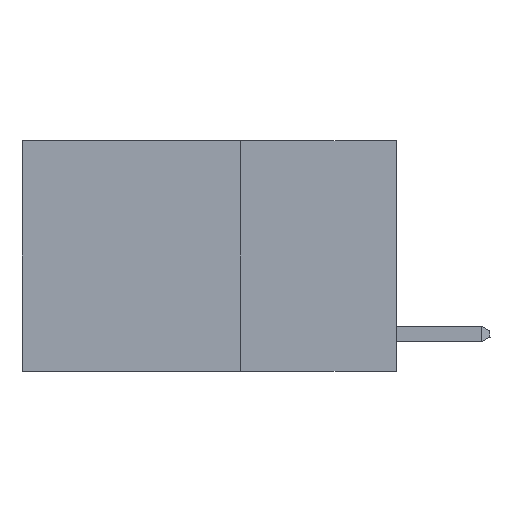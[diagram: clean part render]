
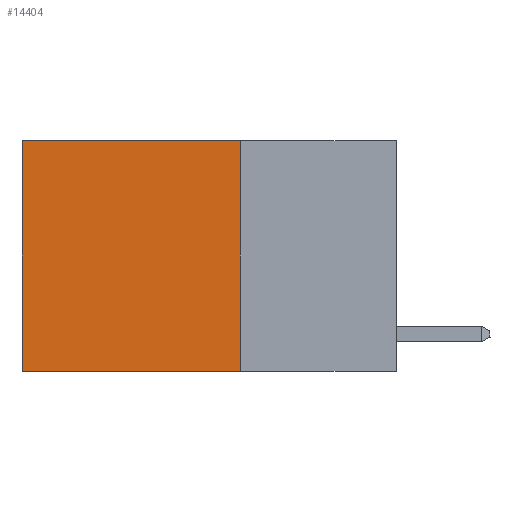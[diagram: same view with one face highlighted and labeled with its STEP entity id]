
A CAD part, left-side view. The second image highlights one B-rep face of the part: STEP entity #14404.
In plain terms, the highlighted planar face has unit normal (-1, 0, 0).
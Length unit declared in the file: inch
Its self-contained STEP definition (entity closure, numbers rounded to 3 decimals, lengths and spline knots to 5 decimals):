
#679 = EDGE_LOOP ( 'NONE', ( #9657, #26297, #12082, #3333 ) ) ;
#1653 = LINE ( 'NONE', #24802, #18273 ) ;
#2124 = VECTOR ( 'NONE', #5819, 39.37008 ) ;
#2194 = CARTESIAN_POINT ( 'NONE',  ( 0.2625, 0.25, 0. ) ) ;
#2763 = LINE ( 'NONE', #22491, #2124 ) ;
#2855 = VERTEX_POINT ( 'NONE', #24447 ) ;
#2958 = EDGE_CURVE ( 'NONE', #21855, #2855, #1653, .T. ) ;
#3333 = ORIENTED_EDGE ( 'NONE', *, *, #18705, .T. ) ;
#3646 = LINE ( 'NONE', #19617, #8541 ) ;
#5655 = EDGE_CURVE ( 'NONE', #2855, #15438, #5745, .T. ) ;
#5745 = LINE ( 'NONE', #22711, #21695 ) ;
#5819 = DIRECTION ( 'NONE',  ( 0., 0., -1. ) ) ;
#6440 = DIRECTION ( 'NONE',  ( 0., 0., -1. ) ) ;
#8541 = VECTOR ( 'NONE', #11299, 39.37008 ) ;
#9657 = ORIENTED_EDGE ( 'NONE', *, *, #17073, .T. ) ;
#11299 = DIRECTION ( 'NONE',  ( 0., 1., 0. ) ) ;
#12082 = ORIENTED_EDGE ( 'NONE', *, *, #2958, .F. ) ;
#12269 = DIRECTION ( 'NONE',  ( 0., 0., -1. ) ) ;
#12712 = CARTESIAN_POINT ( 'NONE',  ( 0.2625, 0.25, 0. ) ) ;
#14404 = ADVANCED_FACE ( 'NONE', ( #15627 ), #16747, .F. ) ;
#15438 = VERTEX_POINT ( 'NONE', #21534 ) ;
#15627 = FACE_OUTER_BOUND ( 'NONE', #679, .T. ) ;
#16358 = DIRECTION ( 'NONE',  ( 0., 1., 0. ) ) ;
#16394 = VERTEX_POINT ( 'NONE', #20496 ) ;
#16747 = PLANE ( 'NONE',  #19987 ) ;
#17073 = EDGE_CURVE ( 'NONE', #16394, #15438, #2763, .T. ) ;
#18273 = VECTOR ( 'NONE', #12269, 39.37008 ) ;
#18705 = EDGE_CURVE ( 'NONE', #21855, #16394, #3646, .T. ) ;
#18878 = DIRECTION ( 'NONE',  ( 1., 0., 0. ) ) ;
#19617 = CARTESIAN_POINT ( 'NONE',  ( 0.2625, 0.25, 0. ) ) ;
#19987 = AXIS2_PLACEMENT_3D ( 'NONE', #2194, #18878, #6440 ) ;
#20496 = CARTESIAN_POINT ( 'NONE',  ( 0.2625, 0.6, 0. ) ) ;
#21534 = CARTESIAN_POINT ( 'NONE',  ( 0.2625, 0.6, -0.37 ) ) ;
#21695 = VECTOR ( 'NONE', #16358, 39.37008 ) ;
#21855 = VERTEX_POINT ( 'NONE', #12712 ) ;
#22491 = CARTESIAN_POINT ( 'NONE',  ( 0.2625, 0.6, 0. ) ) ;
#22711 = CARTESIAN_POINT ( 'NONE',  ( 0.2625, 0.25, -0.37 ) ) ;
#24447 = CARTESIAN_POINT ( 'NONE',  ( 0.2625, 0.25, -0.37 ) ) ;
#24802 = CARTESIAN_POINT ( 'NONE',  ( 0.2625, 0.25, 0. ) ) ;
#26297 = ORIENTED_EDGE ( 'NONE', *, *, #5655, .F. ) ;
